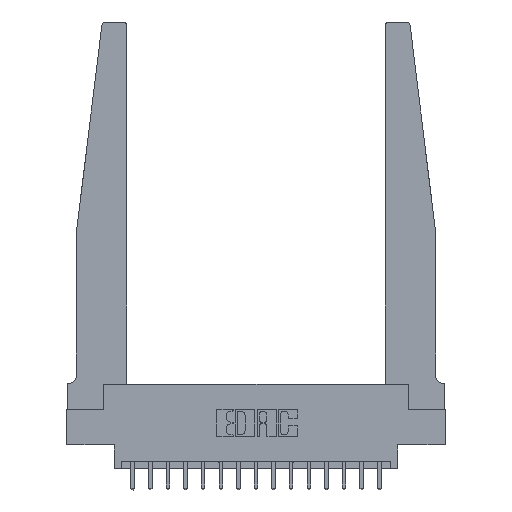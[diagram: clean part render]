
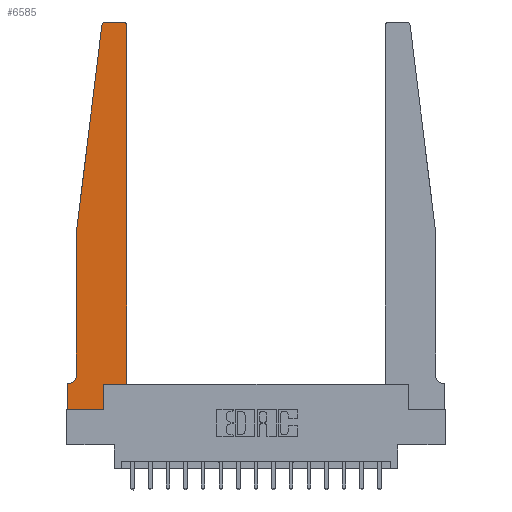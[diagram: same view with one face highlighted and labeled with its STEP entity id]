
A CAD part, top view. The second image highlights one B-rep face of the part: STEP entity #6585.
In plain terms, the highlighted planar face has unit normal (0, 0, 1).
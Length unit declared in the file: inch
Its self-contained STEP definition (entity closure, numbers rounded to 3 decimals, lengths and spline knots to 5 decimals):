
#216 = LINE ( 'NONE', #7223, #7873 ) ;
#476 = VECTOR ( 'NONE', #12046, 39.37008 ) ;
#663 = CARTESIAN_POINT ( 'NONE',  ( 0.015, 0.1875, 0.37 ) ) ;
#679 = VECTOR ( 'NONE', #9899, 39.37008 ) ;
#1026 = EDGE_CURVE ( 'NONE', #15876, #5904, #13442, .T. ) ;
#1151 = CARTESIAN_POINT ( 'NONE',  ( 0.065, 1.25, 0.37 ) ) ;
#1284 = LINE ( 'NONE', #16493, #12221 ) ;
#1334 = CARTESIAN_POINT ( 'NONE',  ( 0., 0., 0.37 ) ) ;
#1411 = EDGE_CURVE ( 'NONE', #9652, #6158, #12056, .T. ) ;
#2348 = CARTESIAN_POINT ( 'NONE',  ( 0.27653, 2.72, 0.37 ) ) ;
#2515 = VECTOR ( 'NONE', #17742, 39.37008 ) ;
#2975 = EDGE_CURVE ( 'NONE', #6349, #6274, #12865, .T. ) ;
#3145 = CARTESIAN_POINT ( 'NONE',  ( 0.425, 2.72, 0.37 ) ) ;
#3394 = ORIENTED_EDGE ( 'NONE', *, *, #1026, .T. ) ;
#3553 = CARTESIAN_POINT ( 'NONE',  ( 0.065, 1.25, 0.37 ) ) ;
#3817 = DIRECTION ( 'NONE',  ( 1., 0., 0. ) ) ;
#3892 = CARTESIAN_POINT ( 'NONE',  ( 0.425, 0.18, 0.37 ) ) ;
#4213 = CIRCLE ( 'NONE', #9706, 0.03 ) ;
#4648 = AXIS2_PLACEMENT_3D ( 'NONE', #2348, #12306, #3817 ) ;
#4672 = VECTOR ( 'NONE', #9009, 39.37008 ) ;
#4857 = DIRECTION ( 'NONE',  ( 0., 0., 1. ) ) ;
#5130 = ORIENTED_EDGE ( 'NONE', *, *, #10451, .T. ) ;
#5300 = VERTEX_POINT ( 'NONE', #8223 ) ;
#5655 = VERTEX_POINT ( 'NONE', #3145 ) ;
#5788 = DIRECTION ( 'NONE',  ( -0.122, -0.992, 0. ) ) ;
#5904 = VERTEX_POINT ( 'NONE', #9598 ) ;
#6158 = VERTEX_POINT ( 'NONE', #15810 ) ;
#6235 = VECTOR ( 'NONE', #7473, 39.37008 ) ;
#6274 = VERTEX_POINT ( 'NONE', #17440 ) ;
#6349 = VERTEX_POINT ( 'NONE', #663 ) ;
#6585 = ADVANCED_FACE ( 'NONE', ( #13648 ), #15311, .T. ) ;
#6639 = VERTEX_POINT ( 'NONE', #1151 ) ;
#6651 = CARTESIAN_POINT ( 'NONE',  ( 0., 0., 0.37 ) ) ;
#6762 = DIRECTION ( 'NONE',  ( 1., 0., 0. ) ) ;
#6880 = DIRECTION ( 'NONE',  ( 0., 0., 1. ) ) ;
#7223 = CARTESIAN_POINT ( 'NONE',  ( 0.065, 1.25, 0.37 ) ) ;
#7232 = AXIS2_PLACEMENT_3D ( 'NONE', #16393, #7986, #17789 ) ;
#7300 = ORIENTED_EDGE ( 'NONE', *, *, #17015, .T. ) ;
#7381 = CIRCLE ( 'NONE', #7232, 0.05 ) ;
#7405 = CARTESIAN_POINT ( 'NONE',  ( 0.24675, 2.72367, 0.37 ) ) ;
#7473 = DIRECTION ( 'NONE',  ( -1., 0., 0. ) ) ;
#7477 = EDGE_CURVE ( 'NONE', #13348, #6639, #216, .T. ) ;
#7482 = CARTESIAN_POINT ( 'NONE',  ( 0.395, 2.75, 0.37 ) ) ;
#7873 = VECTOR ( 'NONE', #5788, 39.37008 ) ;
#7986 = DIRECTION ( 'NONE',  ( 0., 0., -1. ) ) ;
#8223 = CARTESIAN_POINT ( 'NONE',  ( 0.065, 0.2375, 0.37 ) ) ;
#8406 = LINE ( 'NONE', #18344, #16317 ) ;
#8436 = LINE ( 'NONE', #14606, #4672 ) ;
#8526 = ORIENTED_EDGE ( 'NONE', *, *, #9002, .T. ) ;
#8936 = AXIS2_PLACEMENT_3D ( 'NONE', #12492, #6880, #16711 ) ;
#9002 = EDGE_CURVE ( 'NONE', #5300, #6349, #7381, .T. ) ;
#9009 = DIRECTION ( 'NONE',  ( -1., 0., 0. ) ) ;
#9328 = CARTESIAN_POINT ( 'NONE',  ( 0.2605, 0.18, 0.37 ) ) ;
#9423 = EDGE_CURVE ( 'NONE', #13647, #12582, #8436, .T. ) ;
#9472 = EDGE_CURVE ( 'NONE', #5655, #13647, #4213, .T. ) ;
#9598 = CARTESIAN_POINT ( 'NONE',  ( 0.425, 0.18, 0.37 ) ) ;
#9652 = VERTEX_POINT ( 'NONE', #6651 ) ;
#9706 = AXIS2_PLACEMENT_3D ( 'NONE', #13330, #4857, #14731 ) ;
#9899 = DIRECTION ( 'NONE',  ( 1., 0., 0. ) ) ;
#10098 = CIRCLE ( 'NONE', #4648, 0.03 ) ;
#10134 = ORIENTED_EDGE ( 'NONE', *, *, #15741, .T. ) ;
#10451 = EDGE_CURVE ( 'NONE', #6274, #9652, #8406, .T. ) ;
#10949 = ORIENTED_EDGE ( 'NONE', *, *, #16635, .T. ) ;
#11293 = CARTESIAN_POINT ( 'NONE',  ( 0.27653, 2.75, 0.37 ) ) ;
#11334 = ORIENTED_EDGE ( 'NONE', *, *, #12307, .T. ) ;
#11642 = CARTESIAN_POINT ( 'NONE',  ( 0.065, 0.1875, 0.37 ) ) ;
#12046 = DIRECTION ( 'NONE',  ( 0., -1., 0. ) ) ;
#12056 = LINE ( 'NONE', #1334, #679 ) ;
#12221 = VECTOR ( 'NONE', #12274, 39.37008 ) ;
#12274 = DIRECTION ( 'NONE',  ( 0., 1., 0. ) ) ;
#12306 = DIRECTION ( 'NONE',  ( 0., 0., 1. ) ) ;
#12307 = EDGE_CURVE ( 'NONE', #12582, #13348, #10098, .T. ) ;
#12492 = CARTESIAN_POINT ( 'NONE',  ( 0., 0.1875, 0.37 ) ) ;
#12582 = VERTEX_POINT ( 'NONE', #11293 ) ;
#12642 = CARTESIAN_POINT ( 'NONE',  ( 0.2605, 0.18, 0.37 ) ) ;
#12865 = LINE ( 'NONE', #11642, #6235 ) ;
#12933 = ORIENTED_EDGE ( 'NONE', *, *, #1411, .T. ) ;
#13330 = CARTESIAN_POINT ( 'NONE',  ( 0.395, 2.72, 0.37 ) ) ;
#13348 = VERTEX_POINT ( 'NONE', #7405 ) ;
#13416 = LINE ( 'NONE', #9328, #2515 ) ;
#13442 = LINE ( 'NONE', #3892, #16706 ) ;
#13647 = VERTEX_POINT ( 'NONE', #7482 ) ;
#13648 = FACE_OUTER_BOUND ( 'NONE', #16732, .T. ) ;
#14606 = CARTESIAN_POINT ( 'NONE',  ( 0.25, 2.75, 0.37 ) ) ;
#14731 = DIRECTION ( 'NONE',  ( 1., 0., 0. ) ) ;
#15135 = LINE ( 'NONE', #3553, #476 ) ;
#15311 = PLANE ( 'NONE',  #8936 ) ;
#15357 = ORIENTED_EDGE ( 'NONE', *, *, #7477, .T. ) ;
#15741 = EDGE_CURVE ( 'NONE', #5904, #5655, #1284, .T. ) ;
#15810 = CARTESIAN_POINT ( 'NONE',  ( 0.2605, 0., 0.37 ) ) ;
#15876 = VERTEX_POINT ( 'NONE', #12642 ) ;
#16317 = VECTOR ( 'NONE', #18286, 39.37008 ) ;
#16393 = CARTESIAN_POINT ( 'NONE',  ( 0.015, 0.2375, 0.37 ) ) ;
#16493 = CARTESIAN_POINT ( 'NONE',  ( 0.425, 0.18, 0.37 ) ) ;
#16635 = EDGE_CURVE ( 'NONE', #6158, #15876, #13416, .T. ) ;
#16706 = VECTOR ( 'NONE', #6762, 39.37008 ) ;
#16711 = DIRECTION ( 'NONE',  ( 1., 0., 0. ) ) ;
#16732 = EDGE_LOOP ( 'NONE', ( #18164, #11334, #15357, #7300, #8526, #18007, #5130, #12933, #10949, #3394, #10134, #17908 ) ) ;
#17015 = EDGE_CURVE ( 'NONE', #6639, #5300, #15135, .T. ) ;
#17440 = CARTESIAN_POINT ( 'NONE',  ( 0., 0.1875, 0.37 ) ) ;
#17742 = DIRECTION ( 'NONE',  ( 0., 1., 0. ) ) ;
#17789 = DIRECTION ( 'NONE',  ( -1., 0., 0. ) ) ;
#17908 = ORIENTED_EDGE ( 'NONE', *, *, #9472, .T. ) ;
#18007 = ORIENTED_EDGE ( 'NONE', *, *, #2975, .T. ) ;
#18164 = ORIENTED_EDGE ( 'NONE', *, *, #9423, .T. ) ;
#18286 = DIRECTION ( 'NONE',  ( 0., -1., 0. ) ) ;
#18344 = CARTESIAN_POINT ( 'NONE',  ( 0., 0., 0.37 ) ) ;
